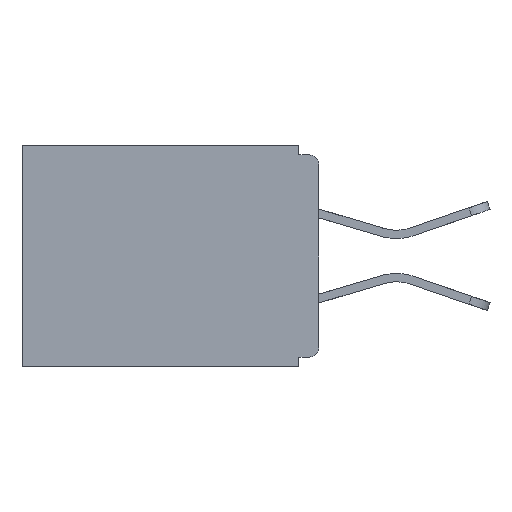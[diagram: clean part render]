
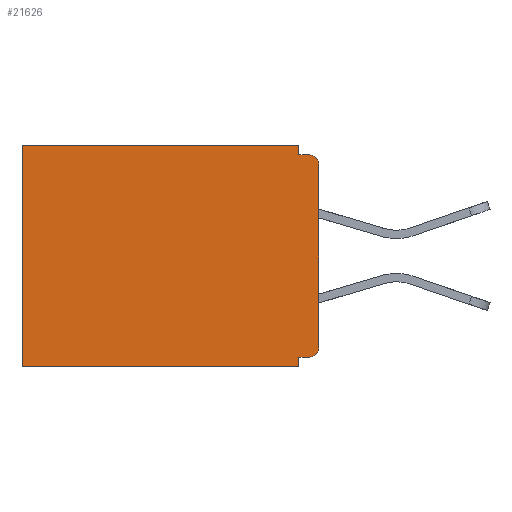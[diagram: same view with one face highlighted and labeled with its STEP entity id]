
A CAD part, left-side view. The second image highlights one B-rep face of the part: STEP entity #21626.
In plain terms, the highlighted planar face has unit normal (-1, 0, 0).
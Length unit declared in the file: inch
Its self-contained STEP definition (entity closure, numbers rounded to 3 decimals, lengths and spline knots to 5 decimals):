
#546 = ORIENTED_EDGE ( 'NONE', *, *, #4553, .F. ) ;
#747 = CARTESIAN_POINT ( 'NONE',  ( 0.298, 0.031, -0.328 ) ) ;
#1003 = VERTEX_POINT ( 'NONE', #6934 ) ;
#1633 = EDGE_CURVE ( 'NONE', #22002, #26469, #23271, .T. ) ;
#1852 = DIRECTION ( 'NONE',  ( 0., 0., -1. ) ) ;
#2252 = CARTESIAN_POINT ( 'NONE',  ( 0.298, 0., 0. ) ) ;
#2742 = DIRECTION ( 'NONE',  ( 0., 1., 0. ) ) ;
#3451 = EDGE_CURVE ( 'NONE', #15906, #3573, #25213, .T. ) ;
#3573 = VERTEX_POINT ( 'NONE', #20518 ) ;
#3987 = EDGE_CURVE ( 'NONE', #22002, #23865, #15119, .T. ) ;
#4045 = EDGE_CURVE ( 'NONE', #15906, #13297, #23119, .T. ) ;
#4106 = VECTOR ( 'NONE', #25171, 39.37008 ) ;
#4223 = DIRECTION ( 'NONE',  ( 0., 0., -1. ) ) ;
#4305 = CARTESIAN_POINT ( 'NONE',  ( 0.298, 0.031, -0.343 ) ) ;
#4553 = EDGE_CURVE ( 'NONE', #23492, #26469, #25157, .T. ) ;
#5126 = VECTOR ( 'NONE', #4223, 39.37008 ) ;
#5131 = ORIENTED_EDGE ( 'NONE', *, *, #3987, .F. ) ;
#5828 = ORIENTED_EDGE ( 'NONE', *, *, #21478, .F. ) ;
#5849 = VECTOR ( 'NONE', #16732, 39.37008 ) ;
#5866 = CIRCLE ( 'NONE', #11966, 0.015 ) ;
#6170 = ORIENTED_EDGE ( 'NONE', *, *, #1633, .T. ) ;
#6934 = CARTESIAN_POINT ( 'NONE',  ( 0.298, 0.46, -0.343 ) ) ;
#7025 = AXIS2_PLACEMENT_3D ( 'NONE', #8473, #19591, #19688 ) ;
#7034 = CARTESIAN_POINT ( 'NONE',  ( 0.298, 0., 0. ) ) ;
#7268 = EDGE_CURVE ( 'NONE', #23492, #14823, #5866, .T. ) ;
#8172 = CARTESIAN_POINT ( 'NONE',  ( 0.298, 0.015, -0.015 ) ) ;
#8473 = CARTESIAN_POINT ( 'NONE',  ( 0.298, 0.015, -0.313 ) ) ;
#8927 = CARTESIAN_POINT ( 'NONE',  ( 0.298, 0.031, -0.015 ) ) ;
#9370 = DIRECTION ( 'NONE',  ( 1., 0., 0. ) ) ;
#9404 = CARTESIAN_POINT ( 'NONE',  ( 0.298, 0., -0.03 ) ) ;
#9573 = CARTESIAN_POINT ( 'NONE',  ( 0.298, 0., -0.343 ) ) ;
#10315 = ORIENTED_EDGE ( 'NONE', *, *, #3451, .T. ) ;
#11272 = CARTESIAN_POINT ( 'NONE',  ( 0.298, 0.031, -0.343 ) ) ;
#11316 = CARTESIAN_POINT ( 'NONE',  ( 0.298, 0.031, 0. ) ) ;
#11426 = VERTEX_POINT ( 'NONE', #11272 ) ;
#11815 = VECTOR ( 'NONE', #21900, 39.37008 ) ;
#11966 = AXIS2_PLACEMENT_3D ( 'NONE', #14884, #23806, #1852 ) ;
#12649 = CARTESIAN_POINT ( 'NONE',  ( 0.298, 0.46, 0. ) ) ;
#12889 = DIRECTION ( 'NONE',  ( 0., 0., -1. ) ) ;
#13297 = VERTEX_POINT ( 'NONE', #8927 ) ;
#13564 = EDGE_CURVE ( 'NONE', #11426, #1003, #25484, .T. ) ;
#13888 = ORIENTED_EDGE ( 'NONE', *, *, #22533, .F. ) ;
#14823 = VERTEX_POINT ( 'NONE', #8172 ) ;
#14884 = CARTESIAN_POINT ( 'NONE',  ( 0.298, 0.015, -0.03 ) ) ;
#15119 = LINE ( 'NONE', #27175, #5849 ) ;
#15183 = DIRECTION ( 'NONE',  ( 0., 0., -1. ) ) ;
#15458 = EDGE_LOOP ( 'NONE', ( #27590, #5828, #18769, #10315, #26888, #27650, #13888, #5131, #6170, #546 ) ) ;
#15536 = FACE_OUTER_BOUND ( 'NONE', #15458, .T. ) ;
#15596 = CARTESIAN_POINT ( 'NONE',  ( 0.298, 0., -0.015 ) ) ;
#15788 = PLANE ( 'NONE',  #16128 ) ;
#15906 = VERTEX_POINT ( 'NONE', #11316 ) ;
#16128 = AXIS2_PLACEMENT_3D ( 'NONE', #7034, #9370, #27187 ) ;
#16192 = VECTOR ( 'NONE', #15183, 39.37008 ) ;
#16388 = CARTESIAN_POINT ( 'NONE',  ( 0.298, 0.031, -0.343 ) ) ;
#16732 = DIRECTION ( 'NONE',  ( 0., 1., 0. ) ) ;
#17219 = VECTOR ( 'NONE', #12889, 39.37008 ) ;
#17246 = VECTOR ( 'NONE', #2742, 39.37008 ) ;
#17264 = LINE ( 'NONE', #12649, #20704 ) ;
#18671 = EDGE_CURVE ( 'NONE', #3573, #1003, #17264, .T. ) ;
#18769 = ORIENTED_EDGE ( 'NONE', *, *, #4045, .F. ) ;
#19591 = DIRECTION ( 'NONE',  ( -1., 0., 0. ) ) ;
#19688 = DIRECTION ( 'NONE',  ( 0., 0., -1. ) ) ;
#20518 = CARTESIAN_POINT ( 'NONE',  ( 0.298, 0.46, 0. ) ) ;
#20704 = VECTOR ( 'NONE', #21298, 39.37008 ) ;
#21298 = DIRECTION ( 'NONE',  ( 0., 0., -1. ) ) ;
#21478 = EDGE_CURVE ( 'NONE', #13297, #14823, #25584, .T. ) ;
#21626 = ADVANCED_FACE ( 'NONE', ( #15536 ), #15788, .F. ) ;
#21900 = DIRECTION ( 'NONE',  ( 0., -1., 0. ) ) ;
#22002 = VERTEX_POINT ( 'NONE', #26408 ) ;
#22081 = LINE ( 'NONE', #16388, #16192 ) ;
#22533 = EDGE_CURVE ( 'NONE', #23865, #11426, #22081, .T. ) ;
#23119 = LINE ( 'NONE', #4305, #17219 ) ;
#23271 = CIRCLE ( 'NONE', #7025, 0.015 ) ;
#23492 = VERTEX_POINT ( 'NONE', #9404 ) ;
#23806 = DIRECTION ( 'NONE',  ( -1., 0., 0. ) ) ;
#23865 = VERTEX_POINT ( 'NONE', #747 ) ;
#24136 = CARTESIAN_POINT ( 'NONE',  ( 0.298, 0., -0.313 ) ) ;
#24725 = CARTESIAN_POINT ( 'NONE',  ( 0.298, 0., 0. ) ) ;
#25157 = LINE ( 'NONE', #2252, #5126 ) ;
#25171 = DIRECTION ( 'NONE',  ( 0., 1., 0. ) ) ;
#25213 = LINE ( 'NONE', #24725, #17246 ) ;
#25484 = LINE ( 'NONE', #9573, #4106 ) ;
#25584 = LINE ( 'NONE', #15596, #11815 ) ;
#26408 = CARTESIAN_POINT ( 'NONE',  ( 0.298, 0.015, -0.328 ) ) ;
#26469 = VERTEX_POINT ( 'NONE', #24136 ) ;
#26888 = ORIENTED_EDGE ( 'NONE', *, *, #18671, .T. ) ;
#27175 = CARTESIAN_POINT ( 'NONE',  ( 0.298, 0., -0.328 ) ) ;
#27187 = DIRECTION ( 'NONE',  ( 0., 0., -1. ) ) ;
#27590 = ORIENTED_EDGE ( 'NONE', *, *, #7268, .T. ) ;
#27650 = ORIENTED_EDGE ( 'NONE', *, *, #13564, .F. ) ;
